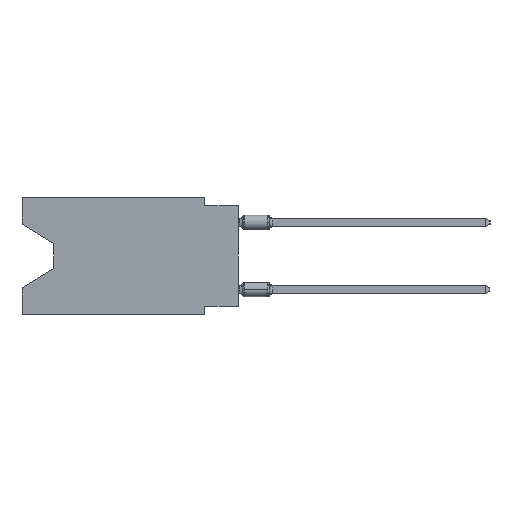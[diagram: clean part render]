
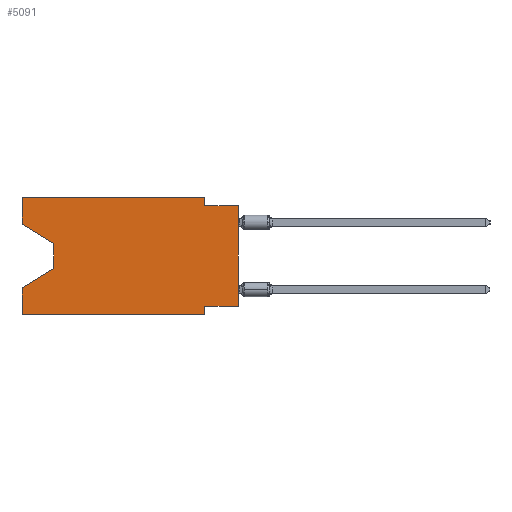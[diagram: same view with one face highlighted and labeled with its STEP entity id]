
A CAD part, left-side view. The second image highlights one B-rep face of the part: STEP entity #5091.
In plain terms, the highlighted planar face has unit normal (-1, 0, 0).
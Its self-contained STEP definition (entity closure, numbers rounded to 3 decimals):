
#270 = DIRECTION ( 'NONE',  ( 0., 0., -1. ) ) ;
#451 = LINE ( 'NONE', #6983, #21154 ) ;
#469 = ORIENTED_EDGE ( 'NONE', *, *, #10744, .F. ) ;
#576 = VERTEX_POINT ( 'NONE', #12304 ) ;
#653 = CARTESIAN_POINT ( 'NONE',  ( 0., 2.54, 0. ) ) ;
#656 = CARTESIAN_POINT ( 'NONE',  ( 0., 16.383, -8.89 ) ) ;
#932 = AXIS2_PLACEMENT_3D ( 'NONE', #18385, #16548, #270 ) ;
#948 = ORIENTED_EDGE ( 'NONE', *, *, #8244, .T. ) ;
#1390 = VERTEX_POINT ( 'NONE', #15079 ) ;
#1632 = EDGE_LOOP ( 'NONE', ( #948, #19959, #4315, #469, #14120, #15541, #5133, #15972, #12491, #13666, #17631, #14999 ) ) ;
#1997 = VECTOR ( 'NONE', #13757, 1000. ) ;
#2297 = EDGE_CURVE ( 'NONE', #20121, #17068, #9034, .T. ) ;
#2301 = VECTOR ( 'NONE', #19856, 1000. ) ;
#3010 = EDGE_CURVE ( 'NONE', #8548, #17123, #17889, .T. ) ;
#3170 = DIRECTION ( 'NONE',  ( 0., -1., 0. ) ) ;
#3273 = VECTOR ( 'NONE', #4532, 1000. ) ;
#3542 = CARTESIAN_POINT ( 'NONE',  ( 0., 0., 0. ) ) ;
#3657 = CARTESIAN_POINT ( 'NONE',  ( 0., 16.383, -8.89 ) ) ;
#4197 = DIRECTION ( 'NONE',  ( 0., 1., 0. ) ) ;
#4315 = ORIENTED_EDGE ( 'NONE', *, *, #14743, .T. ) ;
#4515 = CARTESIAN_POINT ( 'NONE',  ( 0., 0., -8.255 ) ) ;
#4532 = DIRECTION ( 'NONE',  ( 0., 0., -1. ) ) ;
#4560 = CARTESIAN_POINT ( 'NONE',  ( 0., 16.383, 0. ) ) ;
#4642 = VERTEX_POINT ( 'NONE', #8866 ) ;
#4846 = VERTEX_POINT ( 'NONE', #12490 ) ;
#5091 = ADVANCED_FACE ( 'NONE', ( #11723 ), #20245, .F. ) ;
#5133 = ORIENTED_EDGE ( 'NONE', *, *, #19506, .F. ) ;
#5388 = VERTEX_POINT ( 'NONE', #3657 ) ;
#5591 = DIRECTION ( 'NONE',  ( 0., 0., 1. ) ) ;
#5938 = CARTESIAN_POINT ( 'NONE',  ( 0., 13.97, -5.385 ) ) ;
#6171 = VERTEX_POINT ( 'NONE', #13894 ) ;
#6316 = VECTOR ( 'NONE', #10090, 1000. ) ;
#6350 = VECTOR ( 'NONE', #15646, 1000. ) ;
#6983 = CARTESIAN_POINT ( 'NONE',  ( 0., 16.383, 0. ) ) ;
#7674 = CARTESIAN_POINT ( 'NONE',  ( 0., 13.97, -3.505 ) ) ;
#8147 = VECTOR ( 'NONE', #9545, 1000. ) ;
#8244 = EDGE_CURVE ( 'NONE', #576, #8548, #19206, .T. ) ;
#8548 = VERTEX_POINT ( 'NONE', #7674 ) ;
#8866 = CARTESIAN_POINT ( 'NONE',  ( 0., 2.54, -8.255 ) ) ;
#9034 = LINE ( 'NONE', #16770, #1997 ) ;
#9111 = DIRECTION ( 'NONE',  ( 0., -1., 0. ) ) ;
#9513 = EDGE_CURVE ( 'NONE', #19652, #11792, #20911, .T. ) ;
#9545 = DIRECTION ( 'NONE',  ( 0., 0., -1. ) ) ;
#9656 = CARTESIAN_POINT ( 'NONE',  ( 0., 13.97, -3.505 ) ) ;
#9915 = EDGE_CURVE ( 'NONE', #11792, #20121, #19243, .T. ) ;
#10090 = DIRECTION ( 'NONE',  ( 0., 0., 1. ) ) ;
#10254 = EDGE_CURVE ( 'NONE', #576, #19652, #451, .T. ) ;
#10725 = CARTESIAN_POINT ( 'NONE',  ( 0., 16.383, -2.038 ) ) ;
#10744 = EDGE_CURVE ( 'NONE', #5388, #4846, #17754, .T. ) ;
#10830 = VECTOR ( 'NONE', #20418, 1000. ) ;
#10903 = CARTESIAN_POINT ( 'NONE',  ( 0., 16.383, 0. ) ) ;
#11590 = LINE ( 'NONE', #3542, #6316 ) ;
#11723 = FACE_OUTER_BOUND ( 'NONE', #1632, .T. ) ;
#11792 = VERTEX_POINT ( 'NONE', #653 ) ;
#11999 = EDGE_CURVE ( 'NONE', #4642, #6171, #12529, .T. ) ;
#12210 = VECTOR ( 'NONE', #3170, 1000. ) ;
#12304 = CARTESIAN_POINT ( 'NONE',  ( 0., 16.383, -2.038 ) ) ;
#12490 = CARTESIAN_POINT ( 'NONE',  ( 0., 16.383, -6.852 ) ) ;
#12491 = ORIENTED_EDGE ( 'NONE', *, *, #2297, .F. ) ;
#12529 = LINE ( 'NONE', #18871, #8147 ) ;
#12763 = LINE ( 'NONE', #4515, #14097 ) ;
#12965 = CARTESIAN_POINT ( 'NONE',  ( 0., 2.54, -0.635 ) ) ;
#13666 = ORIENTED_EDGE ( 'NONE', *, *, #9915, .F. ) ;
#13757 = DIRECTION ( 'NONE',  ( 0., -1., 0. ) ) ;
#13894 = CARTESIAN_POINT ( 'NONE',  ( 0., 2.54, -8.89 ) ) ;
#13957 = LINE ( 'NONE', #18676, #10830 ) ;
#14097 = VECTOR ( 'NONE', #4197, 1000. ) ;
#14120 = ORIENTED_EDGE ( 'NONE', *, *, #15279, .T. ) ;
#14743 = EDGE_CURVE ( 'NONE', #17123, #4846, #13957, .T. ) ;
#14999 = ORIENTED_EDGE ( 'NONE', *, *, #10254, .F. ) ;
#15079 = CARTESIAN_POINT ( 'NONE',  ( 0., 0., -8.255 ) ) ;
#15279 = EDGE_CURVE ( 'NONE', #5388, #6171, #15330, .T. ) ;
#15284 = VECTOR ( 'NONE', #19372, 1000. ) ;
#15330 = LINE ( 'NONE', #656, #15856 ) ;
#15541 = ORIENTED_EDGE ( 'NONE', *, *, #11999, .F. ) ;
#15646 = DIRECTION ( 'NONE',  ( 0., -0.855, -0.519 ) ) ;
#15856 = VECTOR ( 'NONE', #9111, 1000. ) ;
#15972 = ORIENTED_EDGE ( 'NONE', *, *, #16401, .T. ) ;
#16113 = CARTESIAN_POINT ( 'NONE',  ( 0., 2.54, 0. ) ) ;
#16401 = EDGE_CURVE ( 'NONE', #1390, #17068, #11590, .T. ) ;
#16548 = DIRECTION ( 'NONE',  ( 1., 0., 0. ) ) ;
#16770 = CARTESIAN_POINT ( 'NONE',  ( 0., 0., -0.635 ) ) ;
#17068 = VERTEX_POINT ( 'NONE', #20342 ) ;
#17123 = VERTEX_POINT ( 'NONE', #5938 ) ;
#17631 = ORIENTED_EDGE ( 'NONE', *, *, #9513, .F. ) ;
#17754 = LINE ( 'NONE', #10903, #15284 ) ;
#17889 = LINE ( 'NONE', #9656, #2301 ) ;
#18385 = CARTESIAN_POINT ( 'NONE',  ( 0., 16.383, 0. ) ) ;
#18676 = CARTESIAN_POINT ( 'NONE',  ( 0., 13.97, -5.385 ) ) ;
#18871 = CARTESIAN_POINT ( 'NONE',  ( 0., 2.54, -8.89 ) ) ;
#19206 = LINE ( 'NONE', #10725, #6350 ) ;
#19243 = LINE ( 'NONE', #16113, #3273 ) ;
#19372 = DIRECTION ( 'NONE',  ( 0., 0., 1. ) ) ;
#19506 = EDGE_CURVE ( 'NONE', #1390, #4642, #12763, .T. ) ;
#19652 = VERTEX_POINT ( 'NONE', #21062 ) ;
#19856 = DIRECTION ( 'NONE',  ( 0., 0., -1. ) ) ;
#19959 = ORIENTED_EDGE ( 'NONE', *, *, #3010, .T. ) ;
#20121 = VERTEX_POINT ( 'NONE', #12965 ) ;
#20245 = PLANE ( 'NONE',  #932 ) ;
#20342 = CARTESIAN_POINT ( 'NONE',  ( 0., 0., -0.635 ) ) ;
#20418 = DIRECTION ( 'NONE',  ( 0., 0.855, -0.519 ) ) ;
#20911 = LINE ( 'NONE', #4560, #12210 ) ;
#21062 = CARTESIAN_POINT ( 'NONE',  ( 0., 16.383, 0. ) ) ;
#21154 = VECTOR ( 'NONE', #5591, 1000. ) ;
